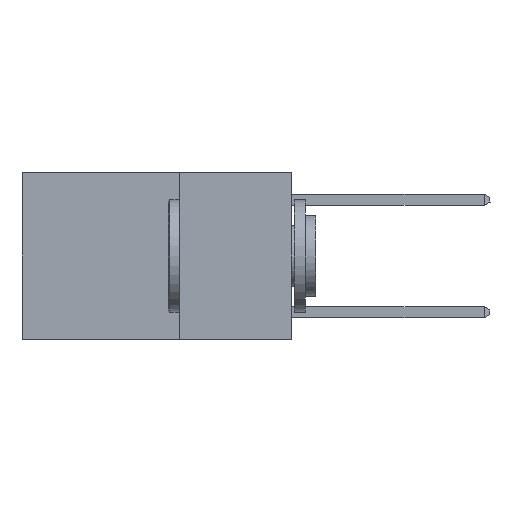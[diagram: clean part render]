
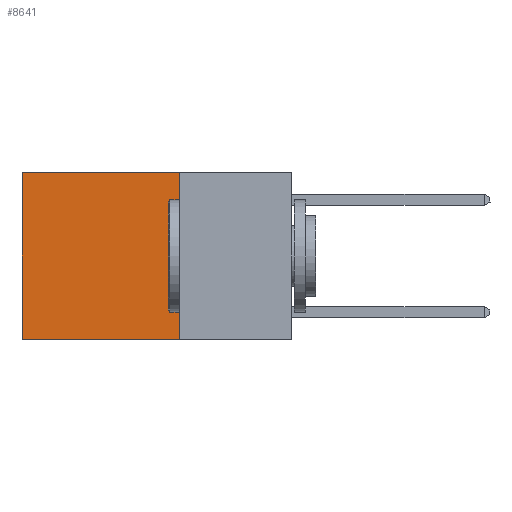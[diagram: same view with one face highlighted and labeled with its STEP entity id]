
A CAD part, left-side view. The second image highlights one B-rep face of the part: STEP entity #8641.
In plain terms, the highlighted planar face has unit normal (-1, 0, 0).
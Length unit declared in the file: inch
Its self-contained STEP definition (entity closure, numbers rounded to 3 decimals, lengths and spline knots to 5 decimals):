
#246 = ORIENTED_EDGE ( 'NONE', *, *, #16047, .T. ) ;
#1712 = CARTESIAN_POINT ( 'NONE',  ( 0.2625, 0.25, -0.37 ) ) ;
#1894 = CARTESIAN_POINT ( 'NONE',  ( 0.2625, 0.6, 0. ) ) ;
#1896 = PLANE ( 'NONE',  #22637 ) ;
#1916 = VERTEX_POINT ( 'NONE', #8585 ) ;
#2325 = EDGE_CURVE ( 'NONE', #1916, #12861, #21777, .T. ) ;
#2901 = VECTOR ( 'NONE', #18570, 39.37008 ) ;
#3899 = CARTESIAN_POINT ( 'NONE',  ( 0.2625, 0.25, 0. ) ) ;
#4474 = CARTESIAN_POINT ( 'NONE',  ( 0.2625, 0.25, 0. ) ) ;
#4531 = CARTESIAN_POINT ( 'NONE',  ( 0.2625, 0.25, -0.37 ) ) ;
#4953 = EDGE_CURVE ( 'NONE', #8091, #12861, #7860, .T. ) ;
#6323 = ORIENTED_EDGE ( 'NONE', *, *, #9929, .F. ) ;
#6509 = DIRECTION ( 'NONE',  ( 0., 1., 0. ) ) ;
#6560 = ORIENTED_EDGE ( 'NONE', *, *, #2325, .T. ) ;
#7839 = VERTEX_POINT ( 'NONE', #4474 ) ;
#7860 = LINE ( 'NONE', #4531, #21041 ) ;
#8087 = LINE ( 'NONE', #19207, #24411 ) ;
#8091 = VERTEX_POINT ( 'NONE', #1712 ) ;
#8244 = DIRECTION ( 'NONE',  ( 0., 0., -1. ) ) ;
#8585 = CARTESIAN_POINT ( 'NONE',  ( 0.2625, 0.6, 0. ) ) ;
#8641 = ADVANCED_FACE ( 'NONE', ( #21649 ), #1896, .F. ) ;
#8701 = VECTOR ( 'NONE', #11739, 39.37008 ) ;
#8964 = EDGE_LOOP ( 'NONE', ( #6560, #19304, #6323, #246 ) ) ;
#9929 = EDGE_CURVE ( 'NONE', #7839, #8091, #8087, .T. ) ;
#11739 = DIRECTION ( 'NONE',  ( 0., 1., 0. ) ) ;
#12861 = VERTEX_POINT ( 'NONE', #17558 ) ;
#13687 = CARTESIAN_POINT ( 'NONE',  ( 0.2625, 0.25, 0. ) ) ;
#14034 = LINE ( 'NONE', #13687, #8701 ) ;
#16047 = EDGE_CURVE ( 'NONE', #7839, #1916, #14034, .T. ) ;
#17558 = CARTESIAN_POINT ( 'NONE',  ( 0.2625, 0.6, -0.37 ) ) ;
#18570 = DIRECTION ( 'NONE',  ( 0., 0., -1. ) ) ;
#19207 = CARTESIAN_POINT ( 'NONE',  ( 0.2625, 0.25, 0. ) ) ;
#19304 = ORIENTED_EDGE ( 'NONE', *, *, #4953, .F. ) ;
#21041 = VECTOR ( 'NONE', #6509, 39.37008 ) ;
#21211 = DIRECTION ( 'NONE',  ( 0., 0., -1. ) ) ;
#21649 = FACE_OUTER_BOUND ( 'NONE', #8964, .T. ) ;
#21777 = LINE ( 'NONE', #1894, #2901 ) ;
#22637 = AXIS2_PLACEMENT_3D ( 'NONE', #3899, #24214, #8244 ) ;
#24214 = DIRECTION ( 'NONE',  ( 1., 0., 0. ) ) ;
#24411 = VECTOR ( 'NONE', #21211, 39.37008 ) ;
